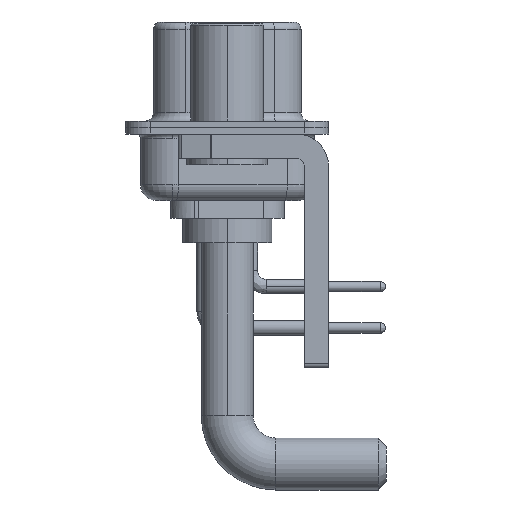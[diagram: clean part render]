
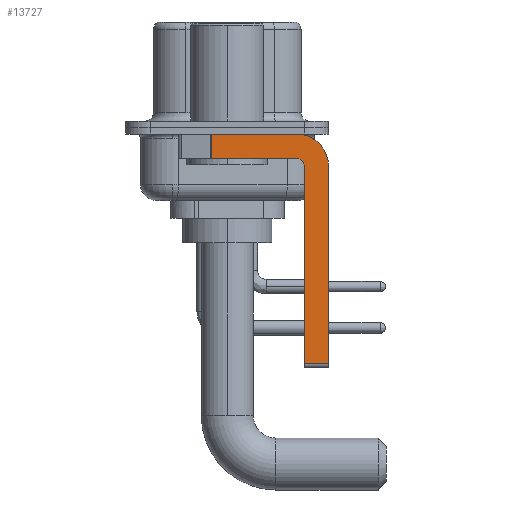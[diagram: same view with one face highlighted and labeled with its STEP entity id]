
A CAD part, left-side view. The second image highlights one B-rep face of the part: STEP entity #13727.
In plain terms, the highlighted planar face has unit normal (-1, 0, 0).
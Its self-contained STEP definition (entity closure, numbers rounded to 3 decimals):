
#265 = CARTESIAN_POINT ( 'NONE',  ( -2.9, -4.25, -2.4 ) ) ;
#888 = ORIENTED_EDGE ( 'NONE', *, *, #9670, .T. ) ;
#1378 = ORIENTED_EDGE ( 'NONE', *, *, #2313, .F. ) ;
#1882 = CARTESIAN_POINT ( 'NONE',  ( -2.9, -4.25, -1.9 ) ) ;
#1937 = VERTEX_POINT ( 'NONE', #14499 ) ;
#2065 = CARTESIAN_POINT ( 'NONE',  ( -2.9, 0.978, -0.4 ) ) ;
#2252 = CARTESIAN_POINT ( 'NONE',  ( -2.9, -6.25, -2.4 ) ) ;
#2313 = EDGE_CURVE ( 'NONE', #1937, #15899, #23664, .T. ) ;
#2540 = VECTOR ( 'NONE', #17861, 1000. ) ;
#3801 = VERTEX_POINT ( 'NONE', #12785 ) ;
#3945 = CARTESIAN_POINT ( 'NONE',  ( -2.9, 3., -0.4 ) ) ;
#4064 = CARTESIAN_POINT ( 'NONE',  ( -2.9, -4.25, -14.55 ) ) ;
#4748 = EDGE_CURVE ( 'NONE', #3801, #18064, #5530, .T. ) ;
#5031 = CARTESIAN_POINT ( 'NONE',  ( -2.9, 0.978, -1.9 ) ) ;
#5475 = VECTOR ( 'NONE', #11878, 1000. ) ;
#5530 = CIRCLE ( 'NONE', #22836, 2. ) ;
#5559 = EDGE_CURVE ( 'NONE', #10068, #23095, #14862, .T. ) ;
#5841 = PLANE ( 'NONE',  #12686 ) ;
#6085 = CARTESIAN_POINT ( 'NONE',  ( -2.9, -6.25, -14.55 ) ) ;
#6087 = LINE ( 'NONE', #3945, #5475 ) ;
#6532 = LINE ( 'NONE', #24067, #7064 ) ;
#7064 = VECTOR ( 'NONE', #12337, 1000. ) ;
#8267 = DIRECTION ( 'NONE',  ( 0., 0., -1. ) ) ;
#8559 = DIRECTION ( 'NONE',  ( 0., 0., -1. ) ) ;
#9110 = VECTOR ( 'NONE', #14444, 1000. ) ;
#9334 = AXIS2_PLACEMENT_3D ( 'NONE', #17613, #23391, #9913 ) ;
#9670 = EDGE_CURVE ( 'NONE', #1937, #18530, #21339, .T. ) ;
#9913 = DIRECTION ( 'NONE',  ( 0., 0., 1. ) ) ;
#9977 = EDGE_CURVE ( 'NONE', #15899, #20267, #10138, .T. ) ;
#10068 = VERTEX_POINT ( 'NONE', #2065 ) ;
#10138 = CIRCLE ( 'NONE', #9334, 0.5 ) ;
#11273 = ORIENTED_EDGE ( 'NONE', *, *, #4748, .F. ) ;
#11351 = ORIENTED_EDGE ( 'NONE', *, *, #5559, .T. ) ;
#11752 = DIRECTION ( 'NONE',  ( 0., -1., 0. ) ) ;
#11878 = DIRECTION ( 'NONE',  ( 0., -1., 0. ) ) ;
#12123 = FACE_OUTER_BOUND ( 'NONE', #13465, .T. ) ;
#12337 = DIRECTION ( 'NONE',  ( 0., 1., 0. ) ) ;
#12686 = AXIS2_PLACEMENT_3D ( 'NONE', #265, #21213, #15672 ) ;
#12785 = CARTESIAN_POINT ( 'NONE',  ( -2.9, -4.25, -0.4 ) ) ;
#13465 = EDGE_LOOP ( 'NONE', ( #23293, #11351, #14618, #22765, #1378, #888, #21931, #11273 ) ) ;
#13727 = ADVANCED_FACE ( 'NONE', ( #12123 ), #5841, .F. ) ;
#13738 = EDGE_CURVE ( 'NONE', #10068, #3801, #6087, .T. ) ;
#13948 = DIRECTION ( 'NONE',  ( 1., 0., 0. ) ) ;
#14311 = CARTESIAN_POINT ( 'NONE',  ( -2.9, -6.25, -2.4 ) ) ;
#14444 = DIRECTION ( 'NONE',  ( 0., 0., -1. ) ) ;
#14499 = CARTESIAN_POINT ( 'NONE',  ( -2.9, -4.75, -14.55 ) ) ;
#14618 = ORIENTED_EDGE ( 'NONE', *, *, #23326, .F. ) ;
#14625 = VECTOR ( 'NONE', #11752, 1000. ) ;
#14688 = LINE ( 'NONE', #14311, #9110 ) ;
#14862 = LINE ( 'NONE', #5031, #23953 ) ;
#15672 = DIRECTION ( 'NONE',  ( 0., 0., -1. ) ) ;
#15899 = VERTEX_POINT ( 'NONE', #22125 ) ;
#15959 = EDGE_CURVE ( 'NONE', #18064, #18530, #14688, .T. ) ;
#17613 = CARTESIAN_POINT ( 'NONE',  ( -2.9, -4.25, -2.4 ) ) ;
#17861 = DIRECTION ( 'NONE',  ( 0., 0., 1. ) ) ;
#18064 = VERTEX_POINT ( 'NONE', #2252 ) ;
#18530 = VERTEX_POINT ( 'NONE', #6085 ) ;
#19751 = CARTESIAN_POINT ( 'NONE',  ( -2.9, -4.25, -2.4 ) ) ;
#19759 = CARTESIAN_POINT ( 'NONE',  ( -2.9, -4.75, -14.8 ) ) ;
#20267 = VERTEX_POINT ( 'NONE', #1882 ) ;
#20442 = CARTESIAN_POINT ( 'NONE',  ( -2.9, 0.978, -1.9 ) ) ;
#21213 = DIRECTION ( 'NONE',  ( 1., 0., 0. ) ) ;
#21339 = LINE ( 'NONE', #4064, #14625 ) ;
#21931 = ORIENTED_EDGE ( 'NONE', *, *, #15959, .F. ) ;
#22125 = CARTESIAN_POINT ( 'NONE',  ( -2.9, -4.75, -2.4 ) ) ;
#22765 = ORIENTED_EDGE ( 'NONE', *, *, #9977, .F. ) ;
#22836 = AXIS2_PLACEMENT_3D ( 'NONE', #19751, #13948, #8267 ) ;
#23095 = VERTEX_POINT ( 'NONE', #20442 ) ;
#23293 = ORIENTED_EDGE ( 'NONE', *, *, #13738, .F. ) ;
#23326 = EDGE_CURVE ( 'NONE', #20267, #23095, #6532, .T. ) ;
#23391 = DIRECTION ( 'NONE',  ( -1., 0., 0. ) ) ;
#23664 = LINE ( 'NONE', #19759, #2540 ) ;
#23953 = VECTOR ( 'NONE', #8559, 1000. ) ;
#24067 = CARTESIAN_POINT ( 'NONE',  ( -2.9, -4.25, -1.9 ) ) ;
